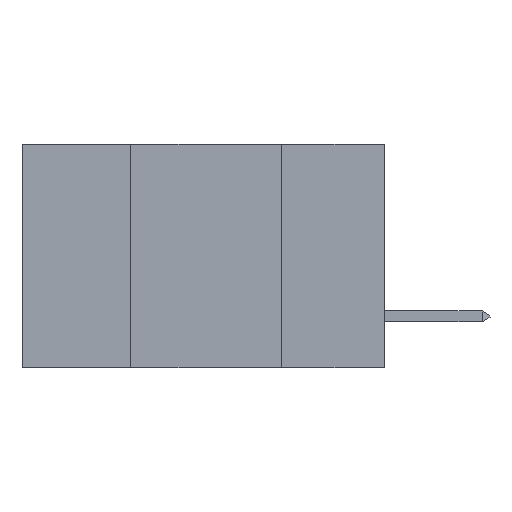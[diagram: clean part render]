
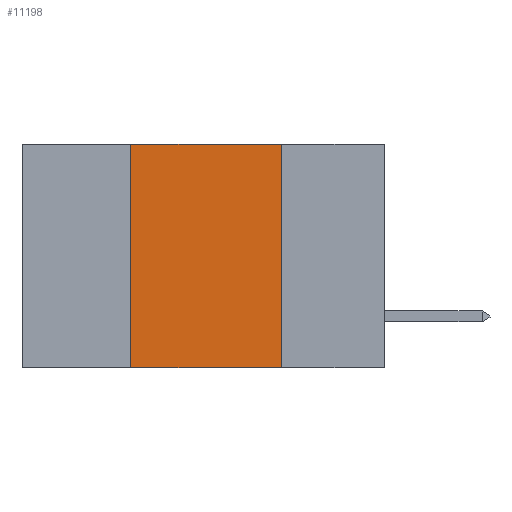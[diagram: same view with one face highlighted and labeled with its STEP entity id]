
A CAD part, left-side view. The second image highlights one B-rep face of the part: STEP entity #11198.
In plain terms, the highlighted planar face has unit normal (-1, 0, 0).
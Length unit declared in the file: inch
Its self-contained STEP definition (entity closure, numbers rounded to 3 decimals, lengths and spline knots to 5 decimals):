
#65 = ORIENTED_EDGE ( 'NONE', *, *, #13791, .F. ) ;
#898 = DIRECTION ( 'NONE',  ( 0., 0., -1. ) ) ;
#1725 = CARTESIAN_POINT ( 'NONE',  ( 0., 0.17, 0. ) ) ;
#2025 = LINE ( 'NONE', #11891, #5933 ) ;
#2404 = CARTESIAN_POINT ( 'NONE',  ( 0., 0.42, -0.37 ) ) ;
#2664 = FACE_OUTER_BOUND ( 'NONE', #8650, .T. ) ;
#2795 = CARTESIAN_POINT ( 'NONE',  ( 0., 0.6, -0.37 ) ) ;
#3501 = AXIS2_PLACEMENT_3D ( 'NONE', #13718, #18947, #898 ) ;
#4259 = LINE ( 'NONE', #2795, #16052 ) ;
#4915 = VERTEX_POINT ( 'NONE', #5360 ) ;
#5110 = ORIENTED_EDGE ( 'NONE', *, *, #12832, .T. ) ;
#5360 = CARTESIAN_POINT ( 'NONE',  ( 0., 0.17, -0.37 ) ) ;
#5827 = VECTOR ( 'NONE', #11648, 39.37008 ) ;
#5933 = VECTOR ( 'NONE', #16714, 39.37008 ) ;
#7459 = EDGE_CURVE ( 'NONE', #11580, #4915, #2025, .T. ) ;
#8650 = EDGE_LOOP ( 'NONE', ( #11060, #65, #21125, #5110 ) ) ;
#10217 = LINE ( 'NONE', #12215, #12809 ) ;
#11060 = ORIENTED_EDGE ( 'NONE', *, *, #7459, .F. ) ;
#11198 = ADVANCED_FACE ( 'NONE', ( #2664 ), #13945, .F. ) ;
#11366 = CARTESIAN_POINT ( 'NONE',  ( 0., 0.6, 0. ) ) ;
#11580 = VERTEX_POINT ( 'NONE', #1725 ) ;
#11648 = DIRECTION ( 'NONE',  ( 0., -1., 0. ) ) ;
#11891 = CARTESIAN_POINT ( 'NONE',  ( 0., 0.17, 0. ) ) ;
#12215 = CARTESIAN_POINT ( 'NONE',  ( 0., 0.42, 0. ) ) ;
#12809 = VECTOR ( 'NONE', #20340, 39.37008 ) ;
#12832 = EDGE_CURVE ( 'NONE', #20564, #4915, #4259, .T. ) ;
#13718 = CARTESIAN_POINT ( 'NONE',  ( 0., 0.6, 0. ) ) ;
#13791 = EDGE_CURVE ( 'NONE', #19912, #11580, #14493, .T. ) ;
#13945 = PLANE ( 'NONE',  #3501 ) ;
#14493 = LINE ( 'NONE', #11366, #5827 ) ;
#16052 = VECTOR ( 'NONE', #19253, 39.37008 ) ;
#16714 = DIRECTION ( 'NONE',  ( 0., 0., -1. ) ) ;
#17544 = CARTESIAN_POINT ( 'NONE',  ( 0., 0.42, 0. ) ) ;
#18947 = DIRECTION ( 'NONE',  ( 1., 0., 0. ) ) ;
#19241 = EDGE_CURVE ( 'NONE', #20564, #19912, #10217, .T. ) ;
#19253 = DIRECTION ( 'NONE',  ( 0., -1., 0. ) ) ;
#19912 = VERTEX_POINT ( 'NONE', #17544 ) ;
#20340 = DIRECTION ( 'NONE',  ( 0., 0., 1. ) ) ;
#20564 = VERTEX_POINT ( 'NONE', #2404 ) ;
#21125 = ORIENTED_EDGE ( 'NONE', *, *, #19241, .F. ) ;
